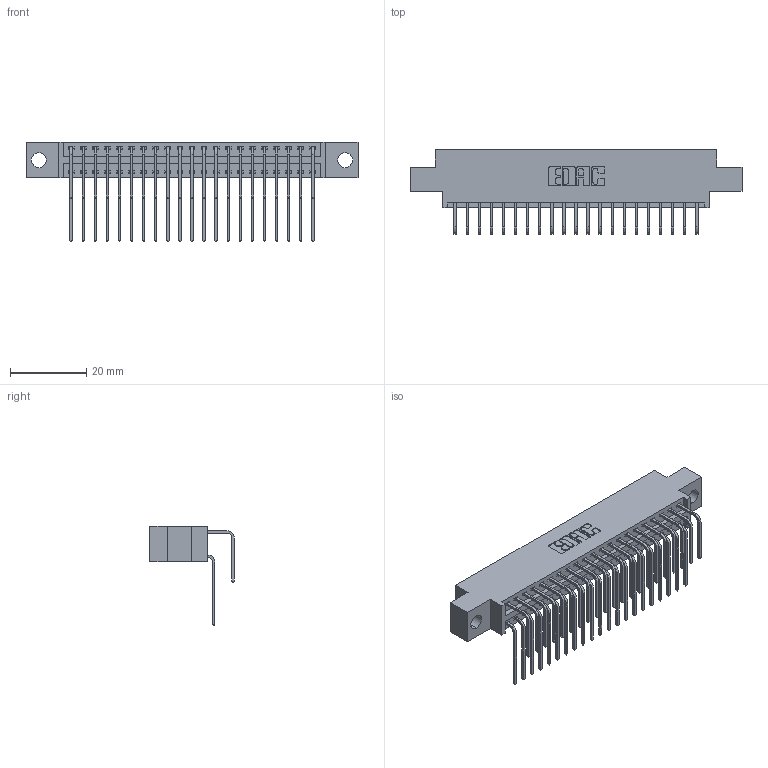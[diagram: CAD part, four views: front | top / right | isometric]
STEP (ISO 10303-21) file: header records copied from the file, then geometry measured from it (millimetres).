
FILE_DESCRIPTION (( 'STEP AP203' ), '1' );
FILE_NAME ('346-042-558-804.STEP', '2022-05-20T05:25:47', ( '' ), ( '' ), 'SwSTEP 2.0', 'SolidWorks 2020', '' );
FILE_SCHEMA (( 'CONFIG_CONTROL_DESIGN' ));
Length unit declared in the file: inch
Products named in the file (4): 346-042-558-804; 346 Part_0.170 Offset - 0.156 Dia-TH; 345-292-001_558 559 Tail - 1; 345-292-001_558 Tail - 2
Assembly tree (43 placements, depth 2):
  346-042-558-804
    346 Part_0.170 Offset - 0.156 Dia-TH
    345-292-001_558 559 Tail - 1  x21
    345-292-001_558 Tail - 2  x21
Bounding box: 87.25 x 22.16 x 26.16 mm (x, y, z)
Volume: 8326.5 mm3; surface area: 12305.1 mm2
Topology: 43 solids, 43 shells, 2408 faces, 7139 edges, 4702 vertices
Faces by surface type: plane 1648, cylinder 760
Entity records: 18867 total; most frequent: CARTESIAN_POINT 3197, ORIENTED_EDGE 3078, DIRECTION 2839, EDGE_CURVE 1539, VECTOR 1283, LINE 1283, VERTEX_POINT 1022, AXIS2_PLACEMENT_3D 778
